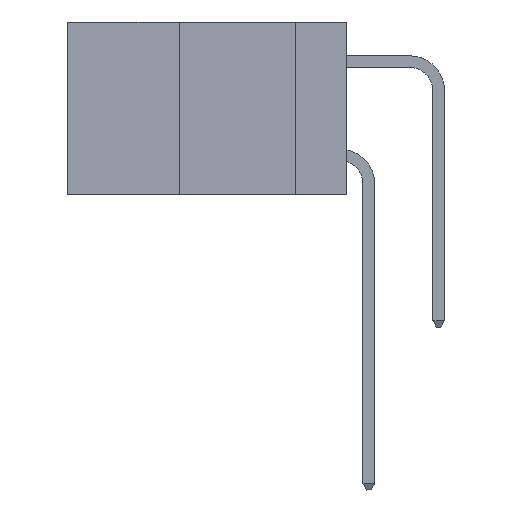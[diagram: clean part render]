
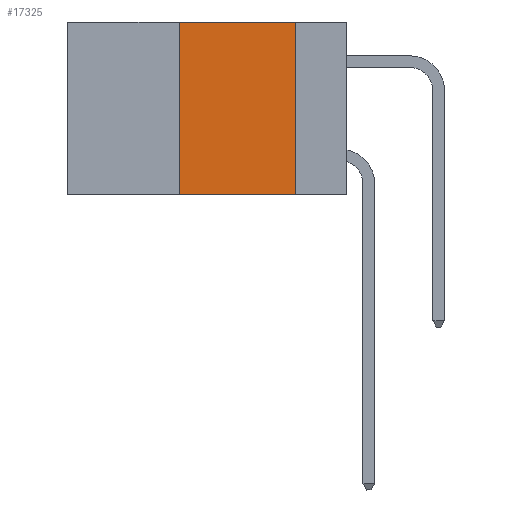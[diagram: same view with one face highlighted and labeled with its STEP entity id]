
A CAD part, left-side view. The second image highlights one B-rep face of the part: STEP entity #17325.
In plain terms, the highlighted planar face has unit normal (-1, 0, 0).
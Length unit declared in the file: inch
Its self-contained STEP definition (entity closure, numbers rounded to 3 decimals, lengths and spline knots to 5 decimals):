
#19 = CARTESIAN_POINT ( 'NONE',  ( 0., 0.11, 0. ) ) ;
#518 = DIRECTION ( 'NONE',  ( 0., 0., -1. ) ) ;
#866 = VERTEX_POINT ( 'NONE', #10978 ) ;
#3444 = CARTESIAN_POINT ( 'NONE',  ( 0., 0.6, 0. ) ) ;
#4120 = CARTESIAN_POINT ( 'NONE',  ( 0., 0.11, -0.37 ) ) ;
#4168 = DIRECTION ( 'NONE',  ( 0., 0., -1. ) ) ;
#4482 = CARTESIAN_POINT ( 'NONE',  ( 0., 0.36, -0.37 ) ) ;
#7116 = ORIENTED_EDGE ( 'NONE', *, *, #27508, .F. ) ;
#10978 = CARTESIAN_POINT ( 'NONE',  ( 0., 0.36, 0. ) ) ;
#11137 = ORIENTED_EDGE ( 'NONE', *, *, #13875, .F. ) ;
#11351 = VECTOR ( 'NONE', #518, 39.37008 ) ;
#12050 = CARTESIAN_POINT ( 'NONE',  ( 0., 0.6, 0. ) ) ;
#12302 = DIRECTION ( 'NONE',  ( 1., 0., 0. ) ) ;
#13875 = EDGE_CURVE ( 'NONE', #31181, #866, #32265, .T. ) ;
#14918 = PLANE ( 'NONE',  #30388 ) ;
#14936 = DIRECTION ( 'NONE',  ( 0., -1., 0. ) ) ;
#17182 = VECTOR ( 'NONE', #22975, 39.37008 ) ;
#17325 = ADVANCED_FACE ( 'NONE', ( #19151 ), #14918, .F. ) ;
#19151 = FACE_OUTER_BOUND ( 'NONE', #19997, .T. ) ;
#19997 = EDGE_LOOP ( 'NONE', ( #32020, #7116, #11137, #33270 ) ) ;
#20720 = VECTOR ( 'NONE', #23555, 39.37008 ) ;
#21040 = CARTESIAN_POINT ( 'NONE',  ( 0., 0.11, 0. ) ) ;
#22975 = DIRECTION ( 'NONE',  ( 0., -1., 0. ) ) ;
#23555 = DIRECTION ( 'NONE',  ( 0., 0., 1. ) ) ;
#24353 = VECTOR ( 'NONE', #14936, 39.37008 ) ;
#24728 = LINE ( 'NONE', #33081, #17182 ) ;
#25418 = VERTEX_POINT ( 'NONE', #21040 ) ;
#27508 = EDGE_CURVE ( 'NONE', #866, #25418, #29250, .T. ) ;
#28657 = EDGE_CURVE ( 'NONE', #25418, #29886, #34015, .T. ) ;
#29022 = CARTESIAN_POINT ( 'NONE',  ( 0., 0.36, 0. ) ) ;
#29250 = LINE ( 'NONE', #3444, #24353 ) ;
#29886 = VERTEX_POINT ( 'NONE', #4120 ) ;
#30388 = AXIS2_PLACEMENT_3D ( 'NONE', #12050, #12302, #4168 ) ;
#31181 = VERTEX_POINT ( 'NONE', #4482 ) ;
#32020 = ORIENTED_EDGE ( 'NONE', *, *, #28657, .F. ) ;
#32265 = LINE ( 'NONE', #29022, #20720 ) ;
#33081 = CARTESIAN_POINT ( 'NONE',  ( 0., 0.6, -0.37 ) ) ;
#33090 = EDGE_CURVE ( 'NONE', #31181, #29886, #24728, .T. ) ;
#33270 = ORIENTED_EDGE ( 'NONE', *, *, #33090, .T. ) ;
#34015 = LINE ( 'NONE', #19, #11351 ) ;
